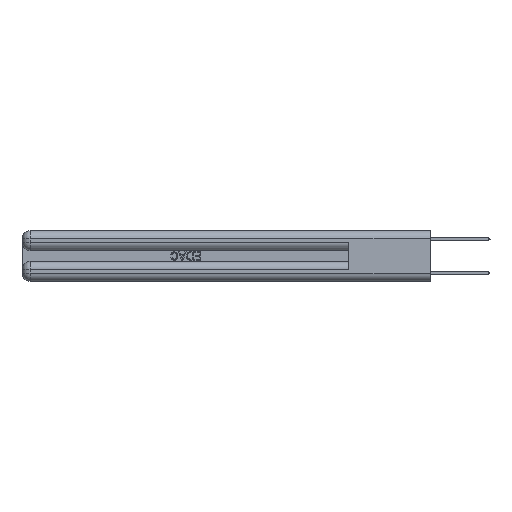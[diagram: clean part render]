
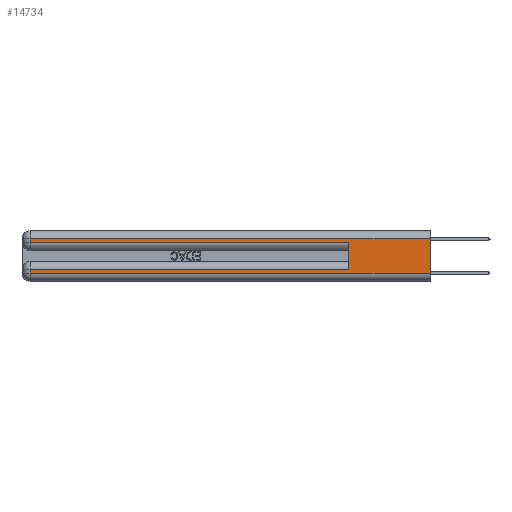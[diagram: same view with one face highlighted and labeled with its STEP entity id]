
A CAD part, left-side view. The second image highlights one B-rep face of the part: STEP entity #14734.
In plain terms, the highlighted planar face has unit normal (-1, 0, 0).
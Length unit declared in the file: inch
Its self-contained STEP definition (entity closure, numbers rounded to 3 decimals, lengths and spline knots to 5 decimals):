
#264 = EDGE_CURVE ( 'NONE', #9948, #14941, #19224, .T. ) ;
#566 = VECTOR ( 'NONE', #26854, 39.37008 ) ;
#568 = EDGE_CURVE ( 'NONE', #8460, #20832, #23463, .T. ) ;
#686 = DIRECTION ( 'NONE',  ( 1., 0., 0. ) ) ;
#1398 = CARTESIAN_POINT ( 'NONE',  ( 0., 0., 0.37 ) ) ;
#1872 = VERTEX_POINT ( 'NONE', #12120 ) ;
#1923 = ORIENTED_EDGE ( 'NONE', *, *, #20131, .T. ) ;
#2011 = ORIENTED_EDGE ( 'NONE', *, *, #9018, .T. ) ;
#2591 = LINE ( 'NONE', #23625, #6403 ) ;
#4391 = ORIENTED_EDGE ( 'NONE', *, *, #10934, .T. ) ;
#5069 = VERTEX_POINT ( 'NONE', #19945 ) ;
#5379 = VECTOR ( 'NONE', #17003, 39.37008 ) ;
#5885 = VECTOR ( 'NONE', #15958, 39.37008 ) ;
#6403 = VECTOR ( 'NONE', #23513, 39.37008 ) ;
#7219 = VERTEX_POINT ( 'NONE', #8267 ) ;
#7294 = VERTEX_POINT ( 'NONE', #15995 ) ;
#8267 = CARTESIAN_POINT ( 'NONE',  ( 0., 2.94, 0.06 ) ) ;
#8342 = VECTOR ( 'NONE', #16324, 39.37008 ) ;
#8460 = VERTEX_POINT ( 'NONE', #20792 ) ;
#9018 = EDGE_CURVE ( 'NONE', #7294, #20832, #21335, .T. ) ;
#9377 = DIRECTION ( 'NONE',  ( 0., -1., 0. ) ) ;
#9948 = VERTEX_POINT ( 'NONE', #25706 ) ;
#10722 = EDGE_CURVE ( 'NONE', #1872, #7219, #2591, .T. ) ;
#10735 = CARTESIAN_POINT ( 'NONE',  ( 0., 0., 0.31 ) ) ;
#10934 = EDGE_CURVE ( 'NONE', #7219, #14941, #22350, .T. ) ;
#11006 = CARTESIAN_POINT ( 'NONE',  ( 0., 0.6, 0.145 ) ) ;
#12120 = CARTESIAN_POINT ( 'NONE',  ( 0., 2.94, 0.085 ) ) ;
#12535 = DIRECTION ( 'NONE',  ( 0., 0., -1. ) ) ;
#12691 = CARTESIAN_POINT ( 'NONE',  ( 0., 0., 0.085 ) ) ;
#13434 = VECTOR ( 'NONE', #9377, 39.37008 ) ;
#13722 = ORIENTED_EDGE ( 'NONE', *, *, #14638, .T. ) ;
#14638 = EDGE_CURVE ( 'NONE', #5069, #7294, #27425, .T. ) ;
#14734 = ADVANCED_FACE ( 'NONE', ( #27050 ), #20870, .F. ) ;
#14941 = VERTEX_POINT ( 'NONE', #23173 ) ;
#15880 = CARTESIAN_POINT ( 'NONE',  ( 0., 0., 0.37 ) ) ;
#15958 = DIRECTION ( 'NONE',  ( 0., 1., 0. ) ) ;
#15995 = CARTESIAN_POINT ( 'NONE',  ( 0., 2.94, 0.285 ) ) ;
#16324 = DIRECTION ( 'NONE',  ( 0., 0., 1. ) ) ;
#17003 = DIRECTION ( 'NONE',  ( 0., -1., 0. ) ) ;
#19224 = LINE ( 'NONE', #1398, #566 ) ;
#19707 = VECTOR ( 'NONE', #12535, 39.37008 ) ;
#19945 = CARTESIAN_POINT ( 'NONE',  ( 0., 2.94, 0.31 ) ) ;
#20131 = EDGE_CURVE ( 'NONE', #9948, #5069, #31533, .T. ) ;
#20767 = DIRECTION ( 'NONE',  ( 0., 0., -1. ) ) ;
#20792 = CARTESIAN_POINT ( 'NONE',  ( 0., 0.6, 0.085 ) ) ;
#20832 = VERTEX_POINT ( 'NONE', #21659 ) ;
#20870 = PLANE ( 'NONE',  #27248 ) ;
#21335 = LINE ( 'NONE', #24053, #5379 ) ;
#21659 = CARTESIAN_POINT ( 'NONE',  ( 0., 0.6, 0.285 ) ) ;
#21801 = ORIENTED_EDGE ( 'NONE', *, *, #10722, .T. ) ;
#22350 = LINE ( 'NONE', #24247, #13434 ) ;
#23173 = CARTESIAN_POINT ( 'NONE',  ( 0., 0., 0.06 ) ) ;
#23463 = LINE ( 'NONE', #11006, #8342 ) ;
#23513 = DIRECTION ( 'NONE',  ( 0., 0., -1. ) ) ;
#23625 = CARTESIAN_POINT ( 'NONE',  ( 0., 2.94, 0.37 ) ) ;
#24053 = CARTESIAN_POINT ( 'NONE',  ( 0., 0., 0.285 ) ) ;
#24247 = CARTESIAN_POINT ( 'NONE',  ( 0., 0., 0.06 ) ) ;
#24744 = EDGE_CURVE ( 'NONE', #8460, #1872, #26972, .T. ) ;
#25706 = CARTESIAN_POINT ( 'NONE',  ( 0., 0., 0.31 ) ) ;
#25947 = ORIENTED_EDGE ( 'NONE', *, *, #568, .F. ) ;
#26854 = DIRECTION ( 'NONE',  ( 0., 0., -1. ) ) ;
#26972 = LINE ( 'NONE', #12691, #27369 ) ;
#27050 = FACE_OUTER_BOUND ( 'NONE', #31964, .T. ) ;
#27248 = AXIS2_PLACEMENT_3D ( 'NONE', #15880, #686, #20767 ) ;
#27344 = CARTESIAN_POINT ( 'NONE',  ( 0., 2.94, 0.37 ) ) ;
#27369 = VECTOR ( 'NONE', #27728, 39.37008 ) ;
#27425 = LINE ( 'NONE', #27344, #19707 ) ;
#27728 = DIRECTION ( 'NONE',  ( 0., 1., 0. ) ) ;
#28064 = ORIENTED_EDGE ( 'NONE', *, *, #264, .F. ) ;
#28560 = ORIENTED_EDGE ( 'NONE', *, *, #24744, .T. ) ;
#31533 = LINE ( 'NONE', #10735, #5885 ) ;
#31964 = EDGE_LOOP ( 'NONE', ( #28064, #1923, #13722, #2011, #25947, #28560, #21801, #4391 ) ) ;
